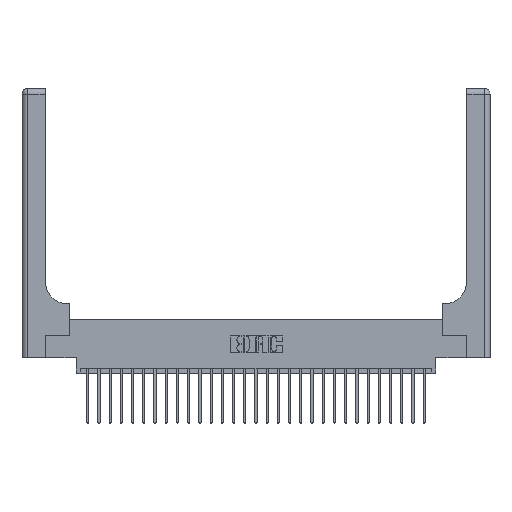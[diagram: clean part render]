
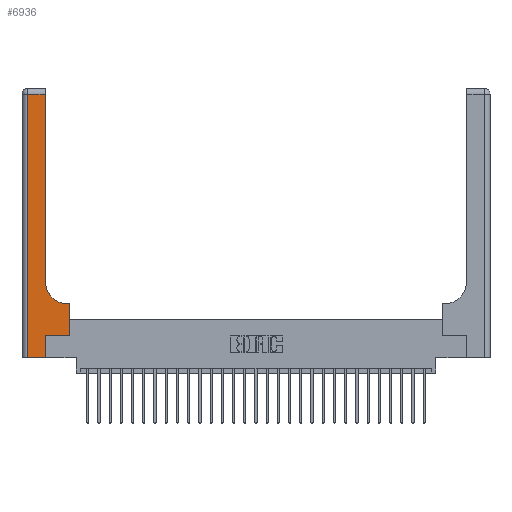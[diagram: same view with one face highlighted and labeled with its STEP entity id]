
A CAD part, top view. The second image highlights one B-rep face of the part: STEP entity #6936.
In plain terms, the highlighted planar face has unit normal (0, 0, 1).
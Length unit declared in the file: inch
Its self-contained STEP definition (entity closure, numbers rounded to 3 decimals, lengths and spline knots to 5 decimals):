
#233 = VECTOR ( 'NONE', #472, 39.37008 ) ;
#472 = DIRECTION ( 'NONE',  ( 0., 1., 0. ) ) ;
#975 = ORIENTED_EDGE ( 'NONE', *, *, #2461, .T. ) ;
#1145 = CARTESIAN_POINT ( 'NONE',  ( 0.26, 0.85, 0.37 ) ) ;
#1270 = PLANE ( 'NONE',  #24567 ) ;
#1458 = VECTOR ( 'NONE', #23460, 39.37008 ) ;
#1460 = DIRECTION ( 'NONE',  ( 1., 0., 0. ) ) ;
#2134 = ORIENTED_EDGE ( 'NONE', *, *, #27246, .T. ) ;
#2140 = ORIENTED_EDGE ( 'NONE', *, *, #17086, .T. ) ;
#2461 = EDGE_CURVE ( 'NONE', #12529, #20183, #15812, .T. ) ;
#2840 = CARTESIAN_POINT ( 'NONE',  ( 0.06, 2.94, 0.37 ) ) ;
#2973 = CARTESIAN_POINT ( 'NONE',  ( 0.26, 2.94, 0.37 ) ) ;
#3292 = DIRECTION ( 'NONE',  ( 0., -1., 0. ) ) ;
#3549 = CARTESIAN_POINT ( 'NONE',  ( 0.51, 0.85, 0.37 ) ) ;
#3649 = EDGE_CURVE ( 'NONE', #14466, #27043, #24096, .T. ) ;
#5021 = ORIENTED_EDGE ( 'NONE', *, *, #13643, .T. ) ;
#6119 = DIRECTION ( 'NONE',  ( 0., 1., 0. ) ) ;
#6264 = VERTEX_POINT ( 'NONE', #24489 ) ;
#6936 = ADVANCED_FACE ( 'NONE', ( #27305 ), #1270, .F. ) ;
#7253 = VECTOR ( 'NONE', #16873, 39.37008 ) ;
#7626 = ORIENTED_EDGE ( 'NONE', *, *, #23473, .T. ) ;
#8098 = VERTEX_POINT ( 'NONE', #2840 ) ;
#8629 = CARTESIAN_POINT ( 'NONE',  ( 0.265, 0.25, 0.37 ) ) ;
#8684 = ORIENTED_EDGE ( 'NONE', *, *, #22110, .T. ) ;
#8985 = LINE ( 'NONE', #17197, #1458 ) ;
#9227 = CARTESIAN_POINT ( 'NONE',  ( 0.26, 3., 0.37 ) ) ;
#9245 = VERTEX_POINT ( 'NONE', #14427 ) ;
#9587 = EDGE_CURVE ( 'NONE', #13633, #8098, #21193, .T. ) ;
#10924 = VECTOR ( 'NONE', #3292, 39.37008 ) ;
#11044 = LINE ( 'NONE', #19534, #12279 ) ;
#11373 = ORIENTED_EDGE ( 'NONE', *, *, #3649, .T. ) ;
#11900 = CARTESIAN_POINT ( 'NONE',  ( 0.265, 0.25, 0.37 ) ) ;
#11904 = LINE ( 'NONE', #20127, #10924 ) ;
#12078 = AXIS2_PLACEMENT_3D ( 'NONE', #3549, #26807, #1460 ) ;
#12279 = VECTOR ( 'NONE', #25951, 39.37008 ) ;
#12395 = DIRECTION ( 'NONE',  ( 0., 0., -1. ) ) ;
#12529 = VERTEX_POINT ( 'NONE', #8629 ) ;
#12992 = LINE ( 'NONE', #18969, #233 ) ;
#13633 = VERTEX_POINT ( 'NONE', #2973 ) ;
#13643 = EDGE_CURVE ( 'NONE', #27043, #13633, #19815, .T. ) ;
#13952 = DIRECTION ( 'NONE',  ( 0., 1., 0. ) ) ;
#14427 = CARTESIAN_POINT ( 'NONE',  ( 0.528, 0.6, 0.37 ) ) ;
#14466 = VERTEX_POINT ( 'NONE', #17982 ) ;
#14518 = VECTOR ( 'NONE', #17891, 39.37008 ) ;
#15812 = LINE ( 'NONE', #11900, #14518 ) ;
#15981 = VERTEX_POINT ( 'NONE', #18828 ) ;
#16425 = LINE ( 'NONE', #16704, #26604 ) ;
#16438 = CARTESIAN_POINT ( 'NONE',  ( 0., 3., 0.37 ) ) ;
#16704 = CARTESIAN_POINT ( 'NONE',  ( 0.265, 0., 0.37 ) ) ;
#16873 = DIRECTION ( 'NONE',  ( -1., 0., 0. ) ) ;
#17086 = EDGE_CURVE ( 'NONE', #9245, #14466, #8985, .T. ) ;
#17197 = CARTESIAN_POINT ( 'NONE',  ( 0.26, 0.6, 0.37 ) ) ;
#17891 = DIRECTION ( 'NONE',  ( 1., 0., 0. ) ) ;
#17982 = CARTESIAN_POINT ( 'NONE',  ( 0.51, 0.6, 0.37 ) ) ;
#18277 = ORIENTED_EDGE ( 'NONE', *, *, #9587, .T. ) ;
#18382 = DIRECTION ( 'NONE',  ( -1., 0., 0. ) ) ;
#18828 = CARTESIAN_POINT ( 'NONE',  ( 0.06, 0., 0.37 ) ) ;
#18969 = CARTESIAN_POINT ( 'NONE',  ( 0.528, 0.25, 0.37 ) ) ;
#19236 = CARTESIAN_POINT ( 'NONE',  ( 0., 2.94, 0.37 ) ) ;
#19534 = CARTESIAN_POINT ( 'NONE',  ( 0., 0., 0.37 ) ) ;
#19815 = LINE ( 'NONE', #9227, #27146 ) ;
#20127 = CARTESIAN_POINT ( 'NONE',  ( 0.06, 3., 0.37 ) ) ;
#20183 = VERTEX_POINT ( 'NONE', #25596 ) ;
#21193 = LINE ( 'NONE', #19236, #7253 ) ;
#21741 = ORIENTED_EDGE ( 'NONE', *, *, #23213, .T. ) ;
#22110 = EDGE_CURVE ( 'NONE', #20183, #9245, #12992, .T. ) ;
#23213 = EDGE_CURVE ( 'NONE', #8098, #15981, #11904, .T. ) ;
#23460 = DIRECTION ( 'NONE',  ( -1., 0., 0. ) ) ;
#23473 = EDGE_CURVE ( 'NONE', #15981, #6264, #11044, .T. ) ;
#23874 = EDGE_LOOP ( 'NONE', ( #5021, #18277, #21741, #7626, #2134, #975, #8684, #2140, #11373 ) ) ;
#24096 = CIRCLE ( 'NONE', #12078, 0.25 ) ;
#24489 = CARTESIAN_POINT ( 'NONE',  ( 0.265, 0., 0.37 ) ) ;
#24567 = AXIS2_PLACEMENT_3D ( 'NONE', #16438, #12395, #18382 ) ;
#25596 = CARTESIAN_POINT ( 'NONE',  ( 0.528, 0.25, 0.37 ) ) ;
#25951 = DIRECTION ( 'NONE',  ( 1., 0., 0. ) ) ;
#26604 = VECTOR ( 'NONE', #6119, 39.37008 ) ;
#26807 = DIRECTION ( 'NONE',  ( 0., 0., -1. ) ) ;
#27043 = VERTEX_POINT ( 'NONE', #1145 ) ;
#27146 = VECTOR ( 'NONE', #13952, 39.37008 ) ;
#27246 = EDGE_CURVE ( 'NONE', #6264, #12529, #16425, .T. ) ;
#27305 = FACE_OUTER_BOUND ( 'NONE', #23874, .T. ) ;
